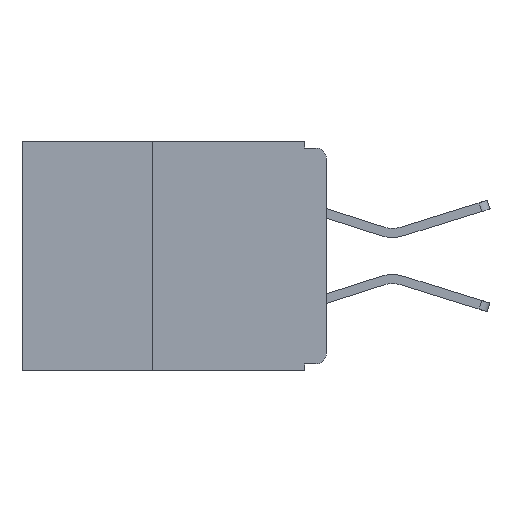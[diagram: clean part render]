
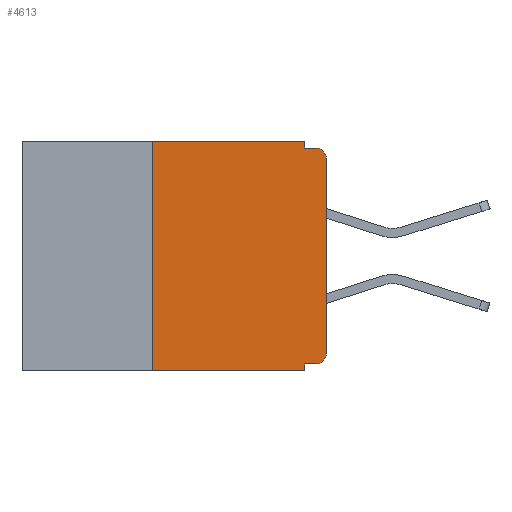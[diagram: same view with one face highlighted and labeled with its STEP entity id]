
A CAD part, left-side view. The second image highlights one B-rep face of the part: STEP entity #4613.
In plain terms, the highlighted planar face has unit normal (-1, 0, 0).
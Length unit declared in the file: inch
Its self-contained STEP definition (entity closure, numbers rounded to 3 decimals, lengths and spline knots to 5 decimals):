
#551 = CARTESIAN_POINT ( 'NONE',  ( 0., 0., -0.025 ) ) ;
#686 = CARTESIAN_POINT ( 'NONE',  ( 0., 0.031, 0. ) ) ;
#830 = VECTOR ( 'NONE', #18225, 39.37008 ) ;
#1088 = EDGE_CURVE ( 'NONE', #16312, #15813, #13385, .T. ) ;
#1164 = VERTEX_POINT ( 'NONE', #551 ) ;
#1240 = VECTOR ( 'NONE', #26000, 39.37008 ) ;
#1278 = CARTESIAN_POINT ( 'NONE',  ( 0., 0.437, -0.33 ) ) ;
#1625 = DIRECTION ( 'NONE',  ( 0., 0., -1. ) ) ;
#1794 = ORIENTED_EDGE ( 'NONE', *, *, #22595, .F. ) ;
#2590 = CARTESIAN_POINT ( 'NONE',  ( 0., 0.015, -0.32 ) ) ;
#3187 = AXIS2_PLACEMENT_3D ( 'NONE', #18565, #5563, #20646 ) ;
#4226 = VECTOR ( 'NONE', #11928, 39.37008 ) ;
#4613 = ADVANCED_FACE ( 'NONE', ( #9114 ), #15625, .F. ) ;
#4908 = VERTEX_POINT ( 'NONE', #9651 ) ;
#5344 = DIRECTION ( 'NONE',  ( 0., -1., 0. ) ) ;
#5563 = DIRECTION ( 'NONE',  ( -1., 0., 0. ) ) ;
#6106 = LINE ( 'NONE', #11860, #26740 ) ;
#6494 = LINE ( 'NONE', #15641, #17388 ) ;
#6901 = ORIENTED_EDGE ( 'NONE', *, *, #21887, .F. ) ;
#7081 = CIRCLE ( 'NONE', #25745, 0.015 ) ;
#7557 = ORIENTED_EDGE ( 'NONE', *, *, #12597, .T. ) ;
#7676 = EDGE_CURVE ( 'NONE', #15813, #11339, #26985, .T. ) ;
#7762 = CARTESIAN_POINT ( 'NONE',  ( 0., 0.015, -0.01 ) ) ;
#8411 = LINE ( 'NONE', #23915, #1240 ) ;
#9114 = FACE_OUTER_BOUND ( 'NONE', #15026, .T. ) ;
#9224 = ORIENTED_EDGE ( 'NONE', *, *, #1088, .F. ) ;
#9531 = AXIS2_PLACEMENT_3D ( 'NONE', #15818, #15515, #15478 ) ;
#9651 = CARTESIAN_POINT ( 'NONE',  ( 0., 0.25, 0. ) ) ;
#9731 = CARTESIAN_POINT ( 'NONE',  ( 0., 0.437, 0. ) ) ;
#10899 = VERTEX_POINT ( 'NONE', #25446 ) ;
#11339 = VERTEX_POINT ( 'NONE', #7762 ) ;
#11860 = CARTESIAN_POINT ( 'NONE',  ( 0., 0., -0.32 ) ) ;
#11928 = DIRECTION ( 'NONE',  ( 0., -1., 0. ) ) ;
#12424 = LINE ( 'NONE', #16076, #830 ) ;
#12597 = EDGE_CURVE ( 'NONE', #17483, #22339, #7081, .T. ) ;
#13002 = ORIENTED_EDGE ( 'NONE', *, *, #19304, .T. ) ;
#13329 = CARTESIAN_POINT ( 'NONE',  ( 0., 0., -0.305 ) ) ;
#13385 = LINE ( 'NONE', #24609, #24650 ) ;
#14664 = DIRECTION ( 'NONE',  ( -1., 0., 0. ) ) ;
#14975 = EDGE_CURVE ( 'NONE', #4908, #16312, #21423, .T. ) ;
#15026 = EDGE_LOOP ( 'NONE', ( #13002, #18760, #20068, #9224, #26830, #16430, #23342, #6901, #1794, #7557 ) ) ;
#15262 = VECTOR ( 'NONE', #24946, 39.37008 ) ;
#15478 = DIRECTION ( 'NONE',  ( 0., 0., -1. ) ) ;
#15515 = DIRECTION ( 'NONE',  ( 1., 0., 0. ) ) ;
#15534 = EDGE_CURVE ( 'NONE', #1164, #11339, #22336, .T. ) ;
#15625 = PLANE ( 'NONE',  #9531 ) ;
#15641 = CARTESIAN_POINT ( 'NONE',  ( 0., 0.031, -0.33 ) ) ;
#15813 = VERTEX_POINT ( 'NONE', #18604 ) ;
#15818 = CARTESIAN_POINT ( 'NONE',  ( 0., 0.437, 0. ) ) ;
#16076 = CARTESIAN_POINT ( 'NONE',  ( 0., 0., 0. ) ) ;
#16312 = VERTEX_POINT ( 'NONE', #686 ) ;
#16430 = ORIENTED_EDGE ( 'NONE', *, *, #24673, .F. ) ;
#17236 = VERTEX_POINT ( 'NONE', #19182 ) ;
#17388 = VECTOR ( 'NONE', #17823, 39.37008 ) ;
#17483 = VERTEX_POINT ( 'NONE', #2590 ) ;
#17823 = DIRECTION ( 'NONE',  ( 0., 0., -1. ) ) ;
#18225 = DIRECTION ( 'NONE',  ( 0., 0., 1. ) ) ;
#18565 = CARTESIAN_POINT ( 'NONE',  ( 0., 0.015, -0.025 ) ) ;
#18604 = CARTESIAN_POINT ( 'NONE',  ( 0., 0.031, -0.01 ) ) ;
#18760 = ORIENTED_EDGE ( 'NONE', *, *, #15534, .T. ) ;
#19182 = CARTESIAN_POINT ( 'NONE',  ( 0., 0.031, -0.32 ) ) ;
#19304 = EDGE_CURVE ( 'NONE', #22339, #1164, #12424, .T. ) ;
#20068 = ORIENTED_EDGE ( 'NONE', *, *, #7676, .F. ) ;
#20646 = DIRECTION ( 'NONE',  ( 0., 0., -1. ) ) ;
#20857 = VECTOR ( 'NONE', #5344, 39.37008 ) ;
#20890 = LINE ( 'NONE', #1278, #15262 ) ;
#21059 = CARTESIAN_POINT ( 'NONE',  ( 0., 0.031, -0.33 ) ) ;
#21423 = LINE ( 'NONE', #9731, #4226 ) ;
#21887 = EDGE_CURVE ( 'NONE', #17236, #25587, #6494, .T. ) ;
#22336 = CIRCLE ( 'NONE', #3187, 0.015 ) ;
#22339 = VERTEX_POINT ( 'NONE', #13329 ) ;
#22532 = CARTESIAN_POINT ( 'NONE',  ( 0., 0., -0.01 ) ) ;
#22595 = EDGE_CURVE ( 'NONE', #17483, #17236, #6106, .T. ) ;
#23301 = EDGE_CURVE ( 'NONE', #10899, #25587, #20890, .T. ) ;
#23342 = ORIENTED_EDGE ( 'NONE', *, *, #23301, .T. ) ;
#23915 = CARTESIAN_POINT ( 'NONE',  ( 0., 0.25, -0.33 ) ) ;
#24552 = DIRECTION ( 'NONE',  ( 0., 0., -1. ) ) ;
#24609 = CARTESIAN_POINT ( 'NONE',  ( 0., 0.031, 0. ) ) ;
#24650 = VECTOR ( 'NONE', #24552, 39.37008 ) ;
#24673 = EDGE_CURVE ( 'NONE', #10899, #4908, #8411, .T. ) ;
#24946 = DIRECTION ( 'NONE',  ( 0., -1., 0. ) ) ;
#25446 = CARTESIAN_POINT ( 'NONE',  ( 0., 0.25, -0.33 ) ) ;
#25587 = VERTEX_POINT ( 'NONE', #21059 ) ;
#25745 = AXIS2_PLACEMENT_3D ( 'NONE', #27193, #14664, #1625 ) ;
#26000 = DIRECTION ( 'NONE',  ( 0., 0., 1. ) ) ;
#26739 = DIRECTION ( 'NONE',  ( 0., 1., 0. ) ) ;
#26740 = VECTOR ( 'NONE', #26739, 39.37008 ) ;
#26830 = ORIENTED_EDGE ( 'NONE', *, *, #14975, .F. ) ;
#26985 = LINE ( 'NONE', #22532, #20857 ) ;
#27193 = CARTESIAN_POINT ( 'NONE',  ( 0., 0.015, -0.305 ) ) ;
